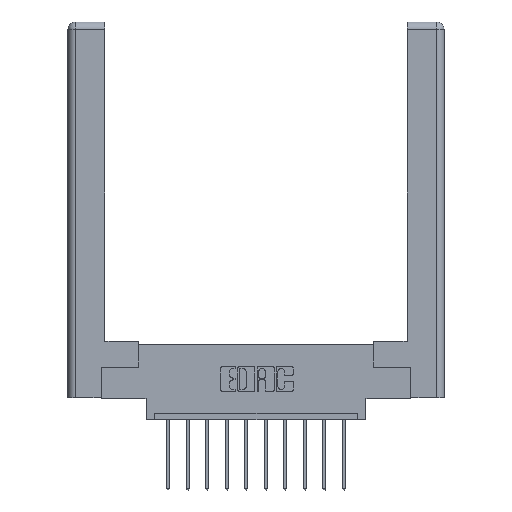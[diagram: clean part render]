
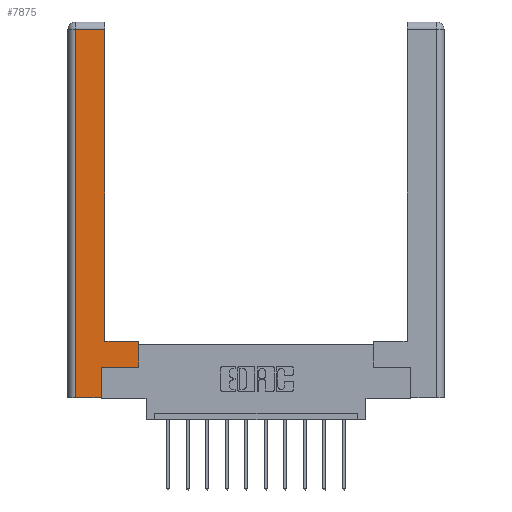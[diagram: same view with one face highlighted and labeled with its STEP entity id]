
A CAD part, top view. The second image highlights one B-rep face of the part: STEP entity #7875.
In plain terms, the highlighted planar face has unit normal (0, 0, 1).
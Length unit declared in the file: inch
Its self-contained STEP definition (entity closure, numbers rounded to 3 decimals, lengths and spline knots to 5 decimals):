
#232 = ORIENTED_EDGE ( 'NONE', *, *, #12496, .T. ) ;
#499 = DIRECTION ( 'NONE',  ( -1., 0., 0. ) ) ;
#511 = VERTEX_POINT ( 'NONE', #2452 ) ;
#708 = ORIENTED_EDGE ( 'NONE', *, *, #10289, .T. ) ;
#822 = EDGE_CURVE ( 'NONE', #4837, #8239, #8262, .T. ) ;
#1723 = DIRECTION ( 'NONE',  ( 1., 0., 0. ) ) ;
#1868 = CARTESIAN_POINT ( 'NONE',  ( 0.0615, 0., 0. ) ) ;
#1917 = ORIENTED_EDGE ( 'NONE', *, *, #9533, .T. ) ;
#2240 = VECTOR ( 'NONE', #12743, 39.37008 ) ;
#2304 = CARTESIAN_POINT ( 'NONE',  ( 0.0615, 2.94, 0. ) ) ;
#2358 = VECTOR ( 'NONE', #12903, 39.37008 ) ;
#2452 = CARTESIAN_POINT ( 'NONE',  ( 0.295, 2.94, 0. ) ) ;
#2577 = VERTEX_POINT ( 'NONE', #10660 ) ;
#2672 = CARTESIAN_POINT ( 'NONE',  ( 0.0615, 2.94, 0. ) ) ;
#2768 = VERTEX_POINT ( 'NONE', #9940 ) ;
#2953 = VERTEX_POINT ( 'NONE', #6673 ) ;
#3447 = ORIENTED_EDGE ( 'NONE', *, *, #12238, .T. ) ;
#3465 = LINE ( 'NONE', #2672, #5557 ) ;
#3921 = LINE ( 'NONE', #5812, #6711 ) ;
#4110 = VECTOR ( 'NONE', #1723, 39.37008 ) ;
#4475 = EDGE_CURVE ( 'NONE', #5765, #2768, #3921, .T. ) ;
#4616 = LINE ( 'NONE', #7190, #6720 ) ;
#4837 = VERTEX_POINT ( 'NONE', #9822 ) ;
#4852 = ORIENTED_EDGE ( 'NONE', *, *, #10327, .T. ) ;
#5086 = DIRECTION ( 'NONE',  ( -1., 0., 0. ) ) ;
#5377 = DIRECTION ( 'NONE',  ( 0., 0., -1. ) ) ;
#5445 = VECTOR ( 'NONE', #7340, 39.37008 ) ;
#5557 = VECTOR ( 'NONE', #11511, 39.37008 ) ;
#5758 = AXIS2_PLACEMENT_3D ( 'NONE', #9469, #5377, #5086 ) ;
#5765 = VERTEX_POINT ( 'NONE', #12774 ) ;
#5812 = CARTESIAN_POINT ( 'NONE',  ( 0.265, 0.245, 0. ) ) ;
#6437 = ORIENTED_EDGE ( 'NONE', *, *, #4475, .T. ) ;
#6673 = CARTESIAN_POINT ( 'NONE',  ( 0.295, 0.45, 0. ) ) ;
#6711 = VECTOR ( 'NONE', #6969, 39.37008 ) ;
#6720 = VECTOR ( 'NONE', #499, 39.37008 ) ;
#6969 = DIRECTION ( 'NONE',  ( 0., 1., 0. ) ) ;
#7130 = CARTESIAN_POINT ( 'NONE',  ( 0.265, 0., 0. ) ) ;
#7190 = CARTESIAN_POINT ( 'NONE',  ( 0.295, 0.45, 0. ) ) ;
#7340 = DIRECTION ( 'NONE',  ( 0., -1., 0. ) ) ;
#7399 = LINE ( 'NONE', #9404, #4110 ) ;
#7875 = ADVANCED_FACE ( 'NONE', ( #12699 ), #13950, .F. ) ;
#8022 = DIRECTION ( 'NONE',  ( 0., 1., 0. ) ) ;
#8221 = VECTOR ( 'NONE', #8022, 39.37008 ) ;
#8239 = VERTEX_POINT ( 'NONE', #9320 ) ;
#8262 = LINE ( 'NONE', #10599, #2358 ) ;
#9092 = CARTESIAN_POINT ( 'NONE',  ( 0.295, 3., 0. ) ) ;
#9320 = CARTESIAN_POINT ( 'NONE',  ( 0.565, 0.45, 0. ) ) ;
#9404 = CARTESIAN_POINT ( 'NONE',  ( 0.565, 0.245, 0. ) ) ;
#9469 = CARTESIAN_POINT ( 'NONE',  ( 0., 0., 0. ) ) ;
#9533 = EDGE_CURVE ( 'NONE', #2577, #5765, #11613, .T. ) ;
#9822 = CARTESIAN_POINT ( 'NONE',  ( 0.565, 0.245, 0. ) ) ;
#9940 = CARTESIAN_POINT ( 'NONE',  ( 0.265, 0.245, 0. ) ) ;
#10289 = EDGE_CURVE ( 'NONE', #2768, #4837, #7399, .T. ) ;
#10327 = EDGE_CURVE ( 'NONE', #8239, #2953, #4616, .T. ) ;
#10599 = CARTESIAN_POINT ( 'NONE',  ( 0.565, 0.45, 0. ) ) ;
#10660 = CARTESIAN_POINT ( 'NONE',  ( 0.0615, 0., 0. ) ) ;
#10731 = ORIENTED_EDGE ( 'NONE', *, *, #13844, .T. ) ;
#11176 = LINE ( 'NONE', #9092, #8221 ) ;
#11511 = DIRECTION ( 'NONE',  ( -1., 0., 0. ) ) ;
#11613 = LINE ( 'NONE', #7130, #2240 ) ;
#12199 = EDGE_LOOP ( 'NONE', ( #232, #10731, #3447, #1917, #6437, #708, #13920, #4852 ) ) ;
#12238 = EDGE_CURVE ( 'NONE', #12500, #2577, #12932, .T. ) ;
#12496 = EDGE_CURVE ( 'NONE', #2953, #511, #11176, .T. ) ;
#12500 = VERTEX_POINT ( 'NONE', #2304 ) ;
#12699 = FACE_OUTER_BOUND ( 'NONE', #12199, .T. ) ;
#12743 = DIRECTION ( 'NONE',  ( 1., 0., 0. ) ) ;
#12774 = CARTESIAN_POINT ( 'NONE',  ( 0.265, 0., 0. ) ) ;
#12903 = DIRECTION ( 'NONE',  ( 0., 1., 0. ) ) ;
#12932 = LINE ( 'NONE', #1868, #5445 ) ;
#13844 = EDGE_CURVE ( 'NONE', #511, #12500, #3465, .T. ) ;
#13920 = ORIENTED_EDGE ( 'NONE', *, *, #822, .T. ) ;
#13950 = PLANE ( 'NONE',  #5758 ) ;
